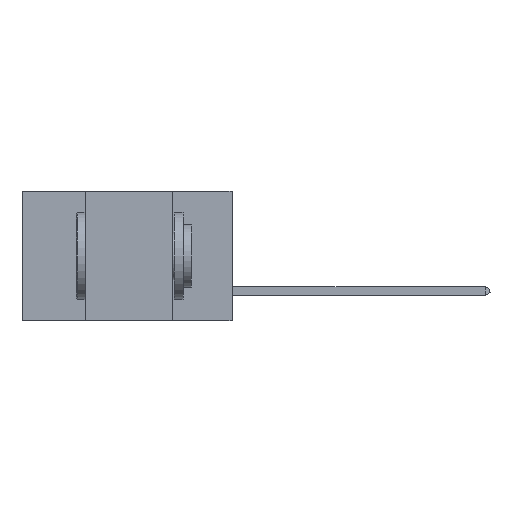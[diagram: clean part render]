
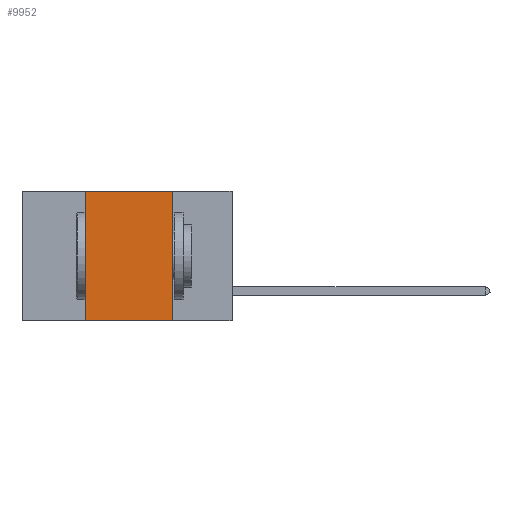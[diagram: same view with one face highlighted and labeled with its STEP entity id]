
A CAD part, left-side view. The second image highlights one B-rep face of the part: STEP entity #9952.
In plain terms, the highlighted planar face has unit normal (-1, 0, 0).
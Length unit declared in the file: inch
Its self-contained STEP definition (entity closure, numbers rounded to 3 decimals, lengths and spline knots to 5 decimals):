
#217 = PLANE ( 'NONE',  #1079 ) ;
#255 = CARTESIAN_POINT ( 'NONE',  ( 0., 0.42, -0.37 ) ) ;
#322 = CARTESIAN_POINT ( 'NONE',  ( 0., 0.6, 0. ) ) ;
#868 = VERTEX_POINT ( 'NONE', #4738 ) ;
#982 = VERTEX_POINT ( 'NONE', #8664 ) ;
#1079 = AXIS2_PLACEMENT_3D ( 'NONE', #322, #3831, #2716 ) ;
#1085 = EDGE_CURVE ( 'NONE', #12475, #11453, #8295, .T. ) ;
#1598 = EDGE_LOOP ( 'NONE', ( #15270, #3523, #14601, #4664 ) ) ;
#1653 = EDGE_CURVE ( 'NONE', #982, #868, #8668, .T. ) ;
#1791 = CARTESIAN_POINT ( 'NONE',  ( 0., 0.17, 0. ) ) ;
#2716 = DIRECTION ( 'NONE',  ( 0., 0., -1. ) ) ;
#2933 = LINE ( 'NONE', #5273, #5526 ) ;
#3523 = ORIENTED_EDGE ( 'NONE', *, *, #4976, .F. ) ;
#3817 = DIRECTION ( 'NONE',  ( 0., 0., 1. ) ) ;
#3831 = DIRECTION ( 'NONE',  ( 1., 0., 0. ) ) ;
#4105 = FACE_OUTER_BOUND ( 'NONE', #1598, .T. ) ;
#4664 = ORIENTED_EDGE ( 'NONE', *, *, #5558, .T. ) ;
#4738 = CARTESIAN_POINT ( 'NONE',  ( 0., 0.17, -0.37 ) ) ;
#4976 = EDGE_CURVE ( 'NONE', #11453, #982, #12309, .T. ) ;
#5273 = CARTESIAN_POINT ( 'NONE',  ( 0., 0.6, -0.37 ) ) ;
#5320 = DIRECTION ( 'NONE',  ( 0., 0., -1. ) ) ;
#5512 = CARTESIAN_POINT ( 'NONE',  ( 0., 0.6, 0. ) ) ;
#5526 = VECTOR ( 'NONE', #12350, 39.37008 ) ;
#5558 = EDGE_CURVE ( 'NONE', #12475, #868, #2933, .T. ) ;
#6475 = VECTOR ( 'NONE', #11832, 39.37008 ) ;
#8295 = LINE ( 'NONE', #14741, #11100 ) ;
#8664 = CARTESIAN_POINT ( 'NONE',  ( 0., 0.17, 0. ) ) ;
#8668 = LINE ( 'NONE', #1791, #11849 ) ;
#9952 = ADVANCED_FACE ( 'NONE', ( #4105 ), #217, .F. ) ;
#11100 = VECTOR ( 'NONE', #3817, 39.37008 ) ;
#11453 = VERTEX_POINT ( 'NONE', #14622 ) ;
#11832 = DIRECTION ( 'NONE',  ( 0., -1., 0. ) ) ;
#11849 = VECTOR ( 'NONE', #5320, 39.37008 ) ;
#12309 = LINE ( 'NONE', #5512, #6475 ) ;
#12350 = DIRECTION ( 'NONE',  ( 0., -1., 0. ) ) ;
#12475 = VERTEX_POINT ( 'NONE', #255 ) ;
#14601 = ORIENTED_EDGE ( 'NONE', *, *, #1085, .F. ) ;
#14622 = CARTESIAN_POINT ( 'NONE',  ( 0., 0.42, 0. ) ) ;
#14741 = CARTESIAN_POINT ( 'NONE',  ( 0., 0.42, 0. ) ) ;
#15270 = ORIENTED_EDGE ( 'NONE', *, *, #1653, .F. ) ;
